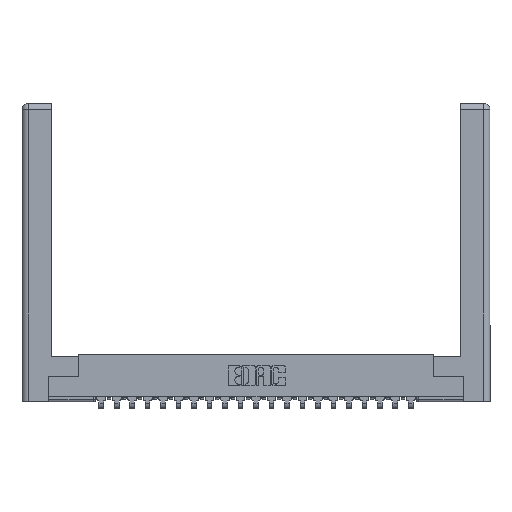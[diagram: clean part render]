
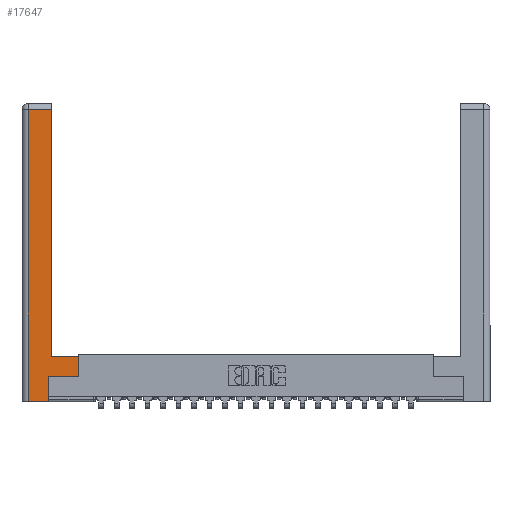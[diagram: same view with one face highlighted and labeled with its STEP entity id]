
A CAD part, top view. The second image highlights one B-rep face of the part: STEP entity #17647.
In plain terms, the highlighted planar face has unit normal (0, 0, 1).
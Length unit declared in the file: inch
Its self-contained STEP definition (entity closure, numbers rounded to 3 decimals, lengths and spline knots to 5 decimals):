
#383 = EDGE_CURVE ( 'NONE', #6707, #8081, #13037, .T. ) ;
#1578 = VERTEX_POINT ( 'NONE', #10268 ) ;
#1959 = LINE ( 'NONE', #11171, #13663 ) ;
#2314 = EDGE_LOOP ( 'NONE', ( #14137, #14249, #2846, #2442, #9800, #2421, #19317, #10535 ) ) ;
#2421 = ORIENTED_EDGE ( 'NONE', *, *, #2618, .T. ) ;
#2442 = ORIENTED_EDGE ( 'NONE', *, *, #383, .T. ) ;
#2580 = CARTESIAN_POINT ( 'NONE',  ( 0.0615, 2.94, 0. ) ) ;
#2618 = EDGE_CURVE ( 'NONE', #8464, #3143, #7894, .T. ) ;
#2783 = CARTESIAN_POINT ( 'NONE',  ( 0.295, 0.45, 0. ) ) ;
#2846 = ORIENTED_EDGE ( 'NONE', *, *, #16480, .T. ) ;
#2948 = DIRECTION ( 'NONE',  ( -1., 0., 0. ) ) ;
#3143 = VERTEX_POINT ( 'NONE', #16721 ) ;
#3257 = VERTEX_POINT ( 'NONE', #2783 ) ;
#3317 = EDGE_CURVE ( 'NONE', #3143, #8011, #16122, .T. ) ;
#4469 = DIRECTION ( 'NONE',  ( 1., 0., 0. ) ) ;
#4832 = DIRECTION ( 'NONE',  ( -1., 0., 0. ) ) ;
#5379 = DIRECTION ( 'NONE',  ( 0., 1., 0. ) ) ;
#5479 = CARTESIAN_POINT ( 'NONE',  ( 0.565, 0.45, 0. ) ) ;
#5770 = VECTOR ( 'NONE', #4832, 39.37008 ) ;
#6647 = CARTESIAN_POINT ( 'NONE',  ( 0.295, 3., 0. ) ) ;
#6707 = VERTEX_POINT ( 'NONE', #20355 ) ;
#6727 = PLANE ( 'NONE',  #12475 ) ;
#6868 = VECTOR ( 'NONE', #11971, 39.37008 ) ;
#7264 = CARTESIAN_POINT ( 'NONE',  ( 0.265, 0.245, 0. ) ) ;
#7894 = LINE ( 'NONE', #16863, #14320 ) ;
#8011 = VERTEX_POINT ( 'NONE', #21808 ) ;
#8081 = VERTEX_POINT ( 'NONE', #11644 ) ;
#8464 = VERTEX_POINT ( 'NONE', #11037 ) ;
#9455 = VECTOR ( 'NONE', #22583, 39.37008 ) ;
#9800 = ORIENTED_EDGE ( 'NONE', *, *, #14026, .T. ) ;
#10248 = EDGE_CURVE ( 'NONE', #8011, #3257, #15374, .T. ) ;
#10268 = CARTESIAN_POINT ( 'NONE',  ( 0.295, 2.94, 0. ) ) ;
#10535 = ORIENTED_EDGE ( 'NONE', *, *, #10248, .T. ) ;
#10666 = LINE ( 'NONE', #6647, #6868 ) ;
#11029 = CARTESIAN_POINT ( 'NONE',  ( 0.265, 0., 0. ) ) ;
#11037 = CARTESIAN_POINT ( 'NONE',  ( 0.265, 0.245, 0. ) ) ;
#11171 = CARTESIAN_POINT ( 'NONE',  ( 0.0615, 0., 0. ) ) ;
#11644 = CARTESIAN_POINT ( 'NONE',  ( 0.265, 0., 0. ) ) ;
#11971 = DIRECTION ( 'NONE',  ( 0., 1., 0. ) ) ;
#12475 = AXIS2_PLACEMENT_3D ( 'NONE', #17362, #17596, #2948 ) ;
#13037 = LINE ( 'NONE', #11029, #14042 ) ;
#13067 = DIRECTION ( 'NONE',  ( 0., -1., 0. ) ) ;
#13663 = VECTOR ( 'NONE', #13067, 39.37008 ) ;
#14026 = EDGE_CURVE ( 'NONE', #8081, #8464, #15012, .T. ) ;
#14042 = VECTOR ( 'NONE', #18333, 39.37008 ) ;
#14137 = ORIENTED_EDGE ( 'NONE', *, *, #18493, .T. ) ;
#14249 = ORIENTED_EDGE ( 'NONE', *, *, #14465, .T. ) ;
#14320 = VECTOR ( 'NONE', #4469, 39.37008 ) ;
#14465 = EDGE_CURVE ( 'NONE', #1578, #21290, #15706, .T. ) ;
#15012 = LINE ( 'NONE', #7264, #18970 ) ;
#15374 = LINE ( 'NONE', #17369, #9455 ) ;
#15492 = VECTOR ( 'NONE', #19788, 39.37008 ) ;
#15706 = LINE ( 'NONE', #2580, #5770 ) ;
#16122 = LINE ( 'NONE', #5479, #15492 ) ;
#16480 = EDGE_CURVE ( 'NONE', #21290, #6707, #1959, .T. ) ;
#16721 = CARTESIAN_POINT ( 'NONE',  ( 0.565, 0.245, 0. ) ) ;
#16863 = CARTESIAN_POINT ( 'NONE',  ( 0.565, 0.245, 0. ) ) ;
#17362 = CARTESIAN_POINT ( 'NONE',  ( 0., 0., 0. ) ) ;
#17369 = CARTESIAN_POINT ( 'NONE',  ( 0.295, 0.45, 0. ) ) ;
#17596 = DIRECTION ( 'NONE',  ( 0., 0., -1. ) ) ;
#17647 = ADVANCED_FACE ( 'NONE', ( #19142 ), #6727, .F. ) ;
#17680 = CARTESIAN_POINT ( 'NONE',  ( 0.0615, 2.94, 0. ) ) ;
#18333 = DIRECTION ( 'NONE',  ( 1., 0., 0. ) ) ;
#18493 = EDGE_CURVE ( 'NONE', #3257, #1578, #10666, .T. ) ;
#18970 = VECTOR ( 'NONE', #5379, 39.37008 ) ;
#19142 = FACE_OUTER_BOUND ( 'NONE', #2314, .T. ) ;
#19317 = ORIENTED_EDGE ( 'NONE', *, *, #3317, .T. ) ;
#19788 = DIRECTION ( 'NONE',  ( 0., 1., 0. ) ) ;
#20355 = CARTESIAN_POINT ( 'NONE',  ( 0.0615, 0., 0. ) ) ;
#21290 = VERTEX_POINT ( 'NONE', #17680 ) ;
#21808 = CARTESIAN_POINT ( 'NONE',  ( 0.565, 0.45, 0. ) ) ;
#22583 = DIRECTION ( 'NONE',  ( -1., 0., 0. ) ) ;
